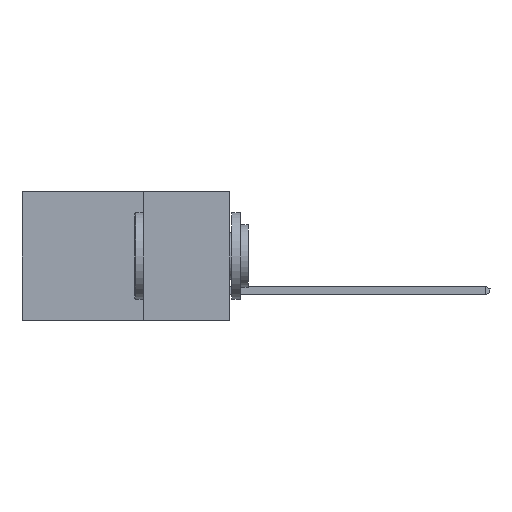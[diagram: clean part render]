
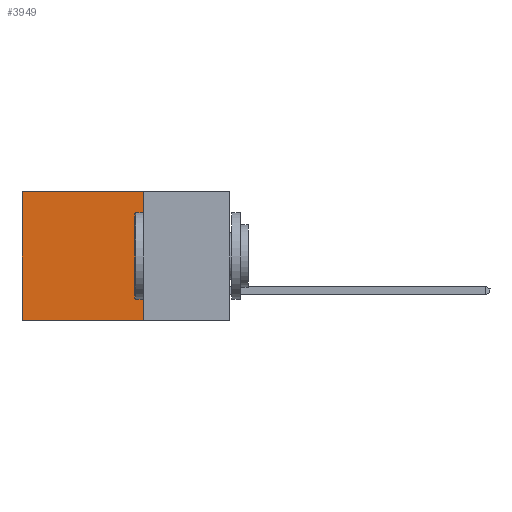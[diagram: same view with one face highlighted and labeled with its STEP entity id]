
A CAD part, left-side view. The second image highlights one B-rep face of the part: STEP entity #3949.
In plain terms, the highlighted planar face has unit normal (-1, 0, 0).
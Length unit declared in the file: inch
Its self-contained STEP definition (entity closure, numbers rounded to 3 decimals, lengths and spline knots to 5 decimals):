
#970 = VECTOR ( 'NONE', #6361, 39.37008 ) ;
#1050 = EDGE_CURVE ( 'NONE', #7055, #12425, #12597, .T. ) ;
#1345 = CARTESIAN_POINT ( 'NONE',  ( 0.2615, 0.25, 0. ) ) ;
#1763 = VERTEX_POINT ( 'NONE', #13979 ) ;
#2554 = DIRECTION ( 'NONE',  ( 0., 1., 0. ) ) ;
#3246 = LINE ( 'NONE', #9586, #12196 ) ;
#3949 = ADVANCED_FACE ( 'NONE', ( #16097 ), #13457, .F. ) ;
#4185 = ORIENTED_EDGE ( 'NONE', *, *, #13564, .F. ) ;
#4715 = DIRECTION ( 'NONE',  ( 0., 0., -1. ) ) ;
#4843 = DIRECTION ( 'NONE',  ( 1., 0., 0. ) ) ;
#6314 = DIRECTION ( 'NONE',  ( 0., 0., -1. ) ) ;
#6361 = DIRECTION ( 'NONE',  ( 0., 1., 0. ) ) ;
#6462 = VECTOR ( 'NONE', #2554, 39.37008 ) ;
#6495 = CARTESIAN_POINT ( 'NONE',  ( 0.2615, 0.25, -0.37 ) ) ;
#7055 = VERTEX_POINT ( 'NONE', #13546 ) ;
#8599 = ORIENTED_EDGE ( 'NONE', *, *, #12001, .F. ) ;
#9230 = CARTESIAN_POINT ( 'NONE',  ( 0.2615, 0.25, -0.37 ) ) ;
#9310 = AXIS2_PLACEMENT_3D ( 'NONE', #12481, #4843, #6314 ) ;
#9336 = VERTEX_POINT ( 'NONE', #15384 ) ;
#9586 = CARTESIAN_POINT ( 'NONE',  ( 0.2615, 0.6, -0.37 ) ) ;
#10681 = EDGE_LOOP ( 'NONE', ( #15242, #4185, #8599, #15813 ) ) ;
#11145 = VECTOR ( 'NONE', #11928, 39.37008 ) ;
#11647 = EDGE_CURVE ( 'NONE', #12425, #9336, #3246, .T. ) ;
#11928 = DIRECTION ( 'NONE',  ( 0., 0., -1. ) ) ;
#12001 = EDGE_CURVE ( 'NONE', #7055, #1763, #13242, .T. ) ;
#12196 = VECTOR ( 'NONE', #4715, 39.37008 ) ;
#12425 = VERTEX_POINT ( 'NONE', #14370 ) ;
#12481 = CARTESIAN_POINT ( 'NONE',  ( 0.2615, 0.25, -0.37 ) ) ;
#12597 = LINE ( 'NONE', #1345, #970 ) ;
#13242 = LINE ( 'NONE', #9230, #11145 ) ;
#13457 = PLANE ( 'NONE',  #9310 ) ;
#13546 = CARTESIAN_POINT ( 'NONE',  ( 0.2615, 0.25, 0. ) ) ;
#13564 = EDGE_CURVE ( 'NONE', #1763, #9336, #14707, .T. ) ;
#13979 = CARTESIAN_POINT ( 'NONE',  ( 0.2615, 0.25, -0.37 ) ) ;
#14370 = CARTESIAN_POINT ( 'NONE',  ( 0.2615, 0.6, 0. ) ) ;
#14707 = LINE ( 'NONE', #6495, #6462 ) ;
#15242 = ORIENTED_EDGE ( 'NONE', *, *, #11647, .T. ) ;
#15384 = CARTESIAN_POINT ( 'NONE',  ( 0.2615, 0.6, -0.37 ) ) ;
#15813 = ORIENTED_EDGE ( 'NONE', *, *, #1050, .T. ) ;
#16097 = FACE_OUTER_BOUND ( 'NONE', #10681, .T. ) ;
